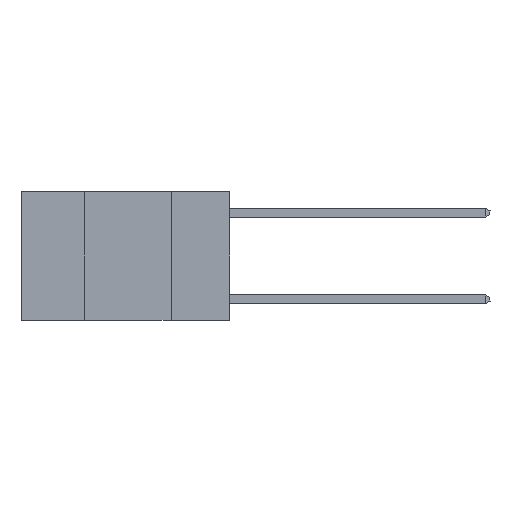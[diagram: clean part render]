
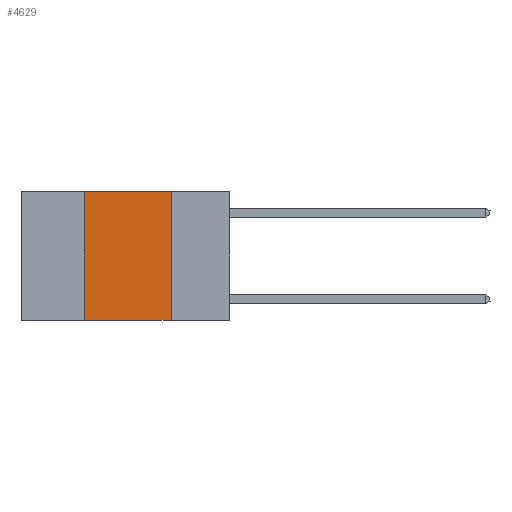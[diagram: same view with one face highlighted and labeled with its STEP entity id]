
A CAD part, left-side view. The second image highlights one B-rep face of the part: STEP entity #4629.
In plain terms, the highlighted planar face has unit normal (-1, 0, 0).
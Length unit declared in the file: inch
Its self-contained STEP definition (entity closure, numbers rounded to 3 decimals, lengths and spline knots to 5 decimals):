
#839 = DIRECTION ( 'NONE',  ( 0., 0., -1. ) ) ;
#1418 = VECTOR ( 'NONE', #5116, 39.37008 ) ;
#4629 = ADVANCED_FACE ( 'NONE', ( #4973 ), #11640, .F. ) ;
#4686 = EDGE_CURVE ( 'NONE', #13497, #27905, #7668, .T. ) ;
#4854 = CARTESIAN_POINT ( 'NONE',  ( 0., 0.17, -0.37 ) ) ;
#4973 = FACE_OUTER_BOUND ( 'NONE', #26017, .T. ) ;
#5116 = DIRECTION ( 'NONE',  ( 0., -1., 0. ) ) ;
#5259 = DIRECTION ( 'NONE',  ( 0., -1., 0. ) ) ;
#5884 = EDGE_CURVE ( 'NONE', #16941, #13497, #26667, .T. ) ;
#6700 = CARTESIAN_POINT ( 'NONE',  ( 0., 0.42, 0. ) ) ;
#7668 = LINE ( 'NONE', #9794, #19768 ) ;
#9311 = EDGE_CURVE ( 'NONE', #19391, #27905, #19860, .T. ) ;
#9794 = CARTESIAN_POINT ( 'NONE',  ( 0., 0.17, 0. ) ) ;
#10217 = VECTOR ( 'NONE', #21433, 39.37008 ) ;
#11018 = ORIENTED_EDGE ( 'NONE', *, *, #4686, .F. ) ;
#11640 = PLANE ( 'NONE',  #19129 ) ;
#12186 = CARTESIAN_POINT ( 'NONE',  ( 0., 0.17, 0. ) ) ;
#13497 = VERTEX_POINT ( 'NONE', #12186 ) ;
#13961 = VECTOR ( 'NONE', #5259, 39.37008 ) ;
#15861 = CARTESIAN_POINT ( 'NONE',  ( 0., 0.6, -0.37 ) ) ;
#15997 = CARTESIAN_POINT ( 'NONE',  ( 0., 0.6, 0. ) ) ;
#16612 = LINE ( 'NONE', #20880, #10217 ) ;
#16941 = VERTEX_POINT ( 'NONE', #6700 ) ;
#18322 = ORIENTED_EDGE ( 'NONE', *, *, #9311, .T. ) ;
#19129 = AXIS2_PLACEMENT_3D ( 'NONE', #15997, #20284, #839 ) ;
#19391 = VERTEX_POINT ( 'NONE', #25637 ) ;
#19768 = VECTOR ( 'NONE', #27345, 39.37008 ) ;
#19860 = LINE ( 'NONE', #15861, #1418 ) ;
#20009 = CARTESIAN_POINT ( 'NONE',  ( 0., 0.6, 0. ) ) ;
#20284 = DIRECTION ( 'NONE',  ( 1., 0., 0. ) ) ;
#20651 = ORIENTED_EDGE ( 'NONE', *, *, #5884, .F. ) ;
#20880 = CARTESIAN_POINT ( 'NONE',  ( 0., 0.42, 0. ) ) ;
#21433 = DIRECTION ( 'NONE',  ( 0., 0., 1. ) ) ;
#22828 = ORIENTED_EDGE ( 'NONE', *, *, #26388, .F. ) ;
#25637 = CARTESIAN_POINT ( 'NONE',  ( 0., 0.42, -0.37 ) ) ;
#26017 = EDGE_LOOP ( 'NONE', ( #11018, #20651, #22828, #18322 ) ) ;
#26388 = EDGE_CURVE ( 'NONE', #19391, #16941, #16612, .T. ) ;
#26667 = LINE ( 'NONE', #20009, #13961 ) ;
#27345 = DIRECTION ( 'NONE',  ( 0., 0., -1. ) ) ;
#27905 = VERTEX_POINT ( 'NONE', #4854 ) ;
